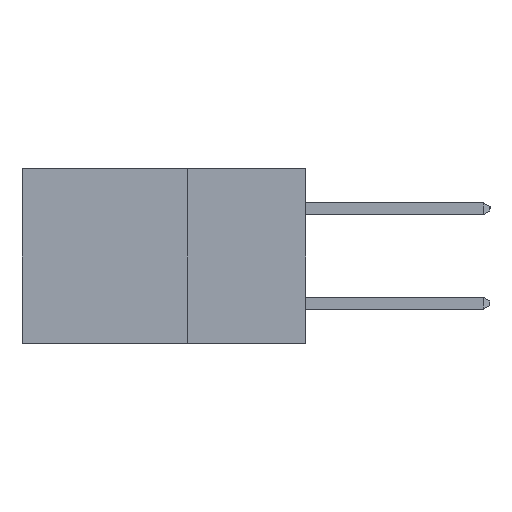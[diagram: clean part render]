
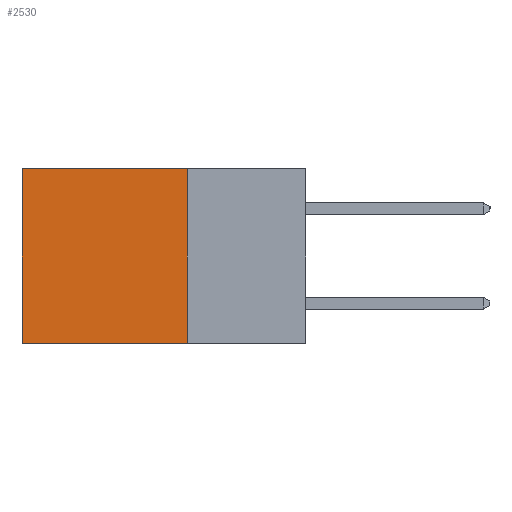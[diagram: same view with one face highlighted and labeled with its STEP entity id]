
A CAD part, left-side view. The second image highlights one B-rep face of the part: STEP entity #2530.
In plain terms, the highlighted planar face has unit normal (-1, 0, 0).
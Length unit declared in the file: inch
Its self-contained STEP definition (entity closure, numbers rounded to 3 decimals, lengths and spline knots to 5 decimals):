
#1072 = FACE_OUTER_BOUND ( 'NONE', #8253, .T. ) ;
#1475 = LINE ( 'NONE', #17634, #19316 ) ;
#1566 = LINE ( 'NONE', #3410, #21977 ) ;
#2053 = CARTESIAN_POINT ( 'NONE',  ( 0.2615, 0.25, 0. ) ) ;
#2530 = ADVANCED_FACE ( 'NONE', ( #1072 ), #11394, .F. ) ;
#2612 = VECTOR ( 'NONE', #11097, 39.37008 ) ;
#3392 = CARTESIAN_POINT ( 'NONE',  ( 0.2615, 0.6, -0.37 ) ) ;
#3410 = CARTESIAN_POINT ( 'NONE',  ( 0.2615, 0.25, -0.37 ) ) ;
#4982 = ORIENTED_EDGE ( 'NONE', *, *, #5108, .F. ) ;
#4996 = VERTEX_POINT ( 'NONE', #6468 ) ;
#5108 = EDGE_CURVE ( 'NONE', #5124, #19068, #1475, .T. ) ;
#5124 = VERTEX_POINT ( 'NONE', #2053 ) ;
#6468 = CARTESIAN_POINT ( 'NONE',  ( 0.2615, 0.6, 0. ) ) ;
#6793 = EDGE_CURVE ( 'NONE', #19068, #9783, #1566, .T. ) ;
#7723 = EDGE_CURVE ( 'NONE', #5124, #4996, #16001, .T. ) ;
#8253 = EDGE_LOOP ( 'NONE', ( #15168, #9259, #4982, #18122 ) ) ;
#8449 = DIRECTION ( 'NONE',  ( 0., 0., -1. ) ) ;
#9259 = ORIENTED_EDGE ( 'NONE', *, *, #6793, .F. ) ;
#9666 = DIRECTION ( 'NONE',  ( 1., 0., 0. ) ) ;
#9783 = VERTEX_POINT ( 'NONE', #3392 ) ;
#11097 = DIRECTION ( 'NONE',  ( 0., 1., 0. ) ) ;
#11394 = PLANE ( 'NONE',  #19225 ) ;
#13764 = DIRECTION ( 'NONE',  ( 0., 1., 0. ) ) ;
#14713 = CARTESIAN_POINT ( 'NONE',  ( 0.2615, 0.25, 0. ) ) ;
#15168 = ORIENTED_EDGE ( 'NONE', *, *, #16719, .T. ) ;
#15240 = CARTESIAN_POINT ( 'NONE',  ( 0.2615, 0.25, -0.37 ) ) ;
#15315 = LINE ( 'NONE', #18813, #21335 ) ;
#15355 = DIRECTION ( 'NONE',  ( 0., 0., -1. ) ) ;
#16001 = LINE ( 'NONE', #14713, #2612 ) ;
#16719 = EDGE_CURVE ( 'NONE', #4996, #9783, #15315, .T. ) ;
#16751 = CARTESIAN_POINT ( 'NONE',  ( 0.2615, 0.25, -0.37 ) ) ;
#17634 = CARTESIAN_POINT ( 'NONE',  ( 0.2615, 0.25, -0.37 ) ) ;
#18122 = ORIENTED_EDGE ( 'NONE', *, *, #7723, .T. ) ;
#18813 = CARTESIAN_POINT ( 'NONE',  ( 0.2615, 0.6, -0.37 ) ) ;
#19046 = DIRECTION ( 'NONE',  ( 0., 0., -1. ) ) ;
#19068 = VERTEX_POINT ( 'NONE', #16751 ) ;
#19225 = AXIS2_PLACEMENT_3D ( 'NONE', #15240, #9666, #15355 ) ;
#19316 = VECTOR ( 'NONE', #8449, 39.37008 ) ;
#21335 = VECTOR ( 'NONE', #19046, 39.37008 ) ;
#21977 = VECTOR ( 'NONE', #13764, 39.37008 ) ;
